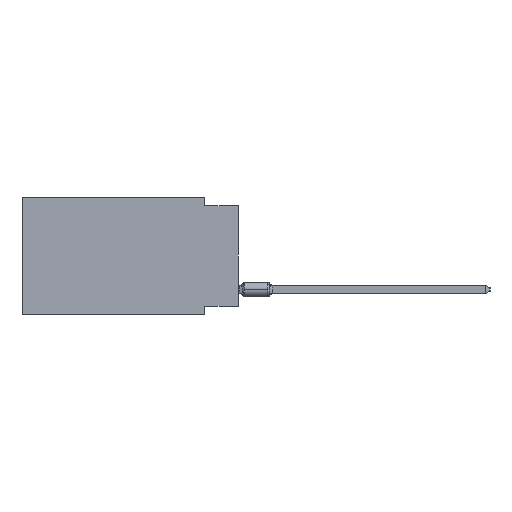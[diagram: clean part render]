
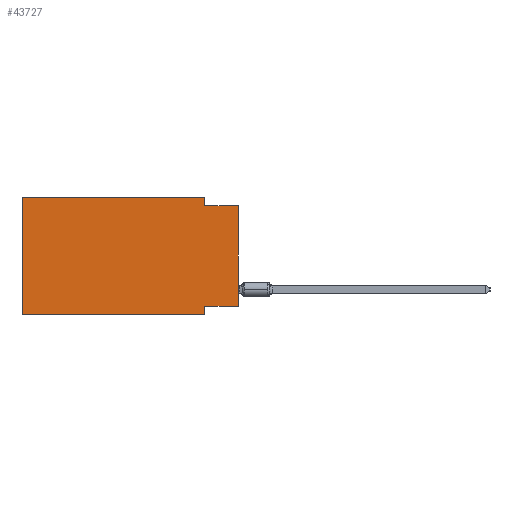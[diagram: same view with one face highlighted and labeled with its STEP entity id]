
A CAD part, left-side view. The second image highlights one B-rep face of the part: STEP entity #43727.
In plain terms, the highlighted planar face has unit normal (-1, 0, 0).
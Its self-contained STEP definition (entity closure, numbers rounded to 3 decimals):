
#2648 = VECTOR ( 'NONE', #24969, 1000. ) ;
#2691 = CARTESIAN_POINT ( 'NONE',  ( 0., 0., -8.255 ) ) ;
#4738 = CARTESIAN_POINT ( 'NONE',  ( 0., 2.54, -8.255 ) ) ;
#5044 = DIRECTION ( 'NONE',  ( 0., -1., 0. ) ) ;
#5581 = LINE ( 'NONE', #26132, #19808 ) ;
#6120 = DIRECTION ( 'NONE',  ( 1., 0., 0. ) ) ;
#6933 = CARTESIAN_POINT ( 'NONE',  ( 0., 2.54, -8.89 ) ) ;
#7012 = DIRECTION ( 'NONE',  ( 0., 0., -1. ) ) ;
#8458 = VERTEX_POINT ( 'NONE', #6933 ) ;
#9522 = VERTEX_POINT ( 'NONE', #34717 ) ;
#9826 = DIRECTION ( 'NONE',  ( 0., 0., 1. ) ) ;
#10451 = PLANE ( 'NONE',  #24901 ) ;
#12033 = ORIENTED_EDGE ( 'NONE', *, *, #22029, .F. ) ;
#12171 = CARTESIAN_POINT ( 'NONE',  ( 0., 0., -8.255 ) ) ;
#13025 = CARTESIAN_POINT ( 'NONE',  ( 0., 16.383, 0. ) ) ;
#13432 = CARTESIAN_POINT ( 'NONE',  ( 0., 16.383, 0. ) ) ;
#13868 = LINE ( 'NONE', #2691, #44936 ) ;
#14022 = VECTOR ( 'NONE', #41219, 1000. ) ;
#15319 = LINE ( 'NONE', #29250, #28796 ) ;
#15944 = CARTESIAN_POINT ( 'NONE',  ( 0., 0., 0. ) ) ;
#16567 = CARTESIAN_POINT ( 'NONE',  ( 0., 2.54, -8.89 ) ) ;
#17132 = LINE ( 'NONE', #13025, #19583 ) ;
#19000 = VERTEX_POINT ( 'NONE', #27726 ) ;
#19057 = EDGE_CURVE ( 'NONE', #39897, #26205, #25189, .T. ) ;
#19583 = VECTOR ( 'NONE', #9826, 1000. ) ;
#19808 = VECTOR ( 'NONE', #40055, 1000. ) ;
#21311 = CARTESIAN_POINT ( 'NONE',  ( 0., 2.54, 0. ) ) ;
#21316 = VECTOR ( 'NONE', #37619, 1000. ) ;
#22029 = EDGE_CURVE ( 'NONE', #26205, #28491, #5581, .T. ) ;
#24151 = ORIENTED_EDGE ( 'NONE', *, *, #38469, .F. ) ;
#24901 = AXIS2_PLACEMENT_3D ( 'NONE', #37395, #6120, #7012 ) ;
#24910 = ORIENTED_EDGE ( 'NONE', *, *, #19057, .F. ) ;
#24969 = DIRECTION ( 'NONE',  ( 0., 0., -1. ) ) ;
#25189 = LINE ( 'NONE', #21311, #2648 ) ;
#26132 = CARTESIAN_POINT ( 'NONE',  ( 0., 0., -0.635 ) ) ;
#26205 = VERTEX_POINT ( 'NONE', #43168 ) ;
#26217 = LINE ( 'NONE', #15944, #30278 ) ;
#27525 = LINE ( 'NONE', #16567, #14022 ) ;
#27726 = CARTESIAN_POINT ( 'NONE',  ( 0., 16.383, 0. ) ) ;
#28054 = EDGE_CURVE ( 'NONE', #9522, #8458, #15319, .T. ) ;
#28414 = EDGE_CURVE ( 'NONE', #34327, #28491, #26217, .T. ) ;
#28491 = VERTEX_POINT ( 'NONE', #43554 ) ;
#28796 = VECTOR ( 'NONE', #5044, 1000. ) ;
#29250 = CARTESIAN_POINT ( 'NONE',  ( 0., 16.383, -8.89 ) ) ;
#29548 = EDGE_CURVE ( 'NONE', #34327, #31211, #13868, .T. ) ;
#30278 = VECTOR ( 'NONE', #36033, 1000. ) ;
#31211 = VERTEX_POINT ( 'NONE', #4738 ) ;
#31477 = ORIENTED_EDGE ( 'NONE', *, *, #35969, .F. ) ;
#31543 = EDGE_LOOP ( 'NONE', ( #42269, #12033, #24910, #39879, #24151, #39471, #31477, #38300 ) ) ;
#32836 = CARTESIAN_POINT ( 'NONE',  ( 0., 2.54, 0. ) ) ;
#34327 = VERTEX_POINT ( 'NONE', #12171 ) ;
#34647 = LINE ( 'NONE', #13432, #21316 ) ;
#34717 = CARTESIAN_POINT ( 'NONE',  ( 0., 16.383, -8.89 ) ) ;
#35969 = EDGE_CURVE ( 'NONE', #31211, #8458, #27525, .T. ) ;
#36033 = DIRECTION ( 'NONE',  ( 0., 0., 1. ) ) ;
#37395 = CARTESIAN_POINT ( 'NONE',  ( 0., 16.383, 0. ) ) ;
#37619 = DIRECTION ( 'NONE',  ( 0., -1., 0. ) ) ;
#38300 = ORIENTED_EDGE ( 'NONE', *, *, #29548, .F. ) ;
#38469 = EDGE_CURVE ( 'NONE', #9522, #19000, #17132, .T. ) ;
#38510 = DIRECTION ( 'NONE',  ( 0., 1., 0. ) ) ;
#39471 = ORIENTED_EDGE ( 'NONE', *, *, #28054, .T. ) ;
#39879 = ORIENTED_EDGE ( 'NONE', *, *, #44815, .F. ) ;
#39897 = VERTEX_POINT ( 'NONE', #32836 ) ;
#40055 = DIRECTION ( 'NONE',  ( 0., -1., 0. ) ) ;
#41219 = DIRECTION ( 'NONE',  ( 0., 0., -1. ) ) ;
#42269 = ORIENTED_EDGE ( 'NONE', *, *, #28414, .T. ) ;
#43168 = CARTESIAN_POINT ( 'NONE',  ( 0., 2.54, -0.635 ) ) ;
#43554 = CARTESIAN_POINT ( 'NONE',  ( 0., 0., -0.635 ) ) ;
#43727 = ADVANCED_FACE ( 'NONE', ( #45143 ), #10451, .F. ) ;
#44815 = EDGE_CURVE ( 'NONE', #19000, #39897, #34647, .T. ) ;
#44936 = VECTOR ( 'NONE', #38510, 1000. ) ;
#45143 = FACE_OUTER_BOUND ( 'NONE', #31543, .T. ) ;
